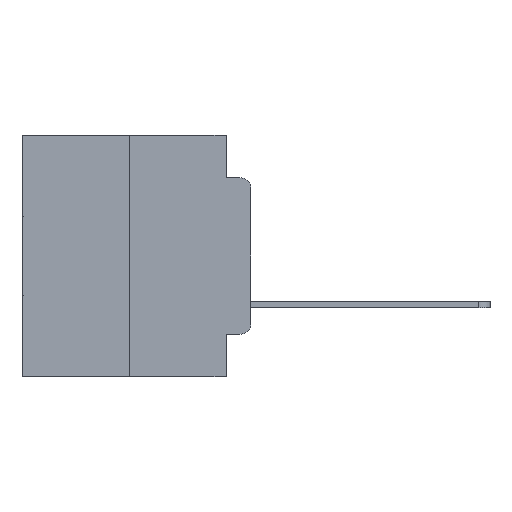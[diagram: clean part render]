
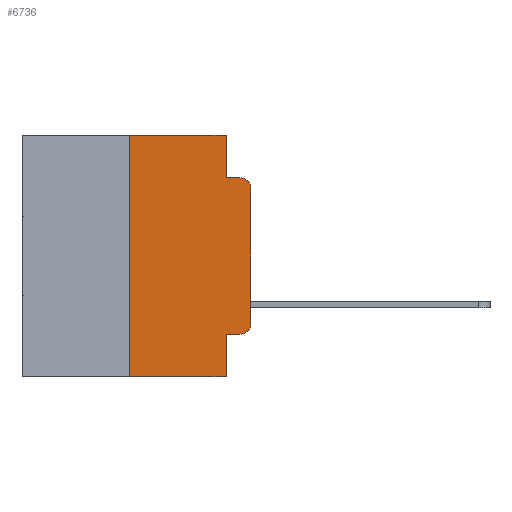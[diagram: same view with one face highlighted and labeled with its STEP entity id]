
A CAD part, left-side view. The second image highlights one B-rep face of the part: STEP entity #6736.
In plain terms, the highlighted planar face has unit normal (-1, 0, 0).
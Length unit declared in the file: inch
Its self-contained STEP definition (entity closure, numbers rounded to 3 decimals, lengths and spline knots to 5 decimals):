
#84 = ORIENTED_EDGE ( 'NONE', *, *, #25238, .F. ) ;
#494 = EDGE_CURVE ( 'NONE', #27528, #16480, #21956, .T. ) ;
#1018 = CARTESIAN_POINT ( 'NONE',  ( 0., 0.02, -0.0885 ) ) ;
#1661 = EDGE_CURVE ( 'NONE', #21829, #10695, #11175, .T. ) ;
#1906 = LINE ( 'NONE', #11384, #2932 ) ;
#2286 = EDGE_LOOP ( 'NONE', ( #9304, #26170, #3473, #11589, #12867, #13742, #19605, #84, #2298, #19662 ) ) ;
#2298 = ORIENTED_EDGE ( 'NONE', *, *, #1661, .T. ) ;
#2320 = LINE ( 'NONE', #20748, #25140 ) ;
#2638 = DIRECTION ( 'NONE',  ( 0., 0., -1. ) ) ;
#2652 = LINE ( 'NONE', #13312, #23407 ) ;
#2932 = VECTOR ( 'NONE', #2638, 39.37008 ) ;
#3473 = ORIENTED_EDGE ( 'NONE', *, *, #16525, .F. ) ;
#3778 = EDGE_CURVE ( 'NONE', #10695, #13114, #21313, .T. ) ;
#4010 = CARTESIAN_POINT ( 'NONE',  ( 0., 0.02, -0.3915 ) ) ;
#4629 = VERTEX_POINT ( 'NONE', #13715 ) ;
#5187 = EDGE_CURVE ( 'NONE', #4629, #9251, #10192, .T. ) ;
#5969 = EDGE_CURVE ( 'NONE', #24840, #12670, #23229, .T. ) ;
#6106 = PLANE ( 'NONE',  #21900 ) ;
#6248 = DIRECTION ( 'NONE',  ( 0., 0., -1. ) ) ;
#6736 = ADVANCED_FACE ( 'NONE', ( #27365 ), #6106, .F. ) ;
#7195 = DIRECTION ( 'NONE',  ( 0., 0., 1. ) ) ;
#7248 = CARTESIAN_POINT ( 'NONE',  ( 0., 0., -0.3915 ) ) ;
#7383 = CARTESIAN_POINT ( 'NONE',  ( 0., 0.25, 0. ) ) ;
#7593 = VECTOR ( 'NONE', #27357, 39.37008 ) ;
#8566 = EDGE_CURVE ( 'NONE', #13114, #27528, #13794, .T. ) ;
#9251 = VERTEX_POINT ( 'NONE', #17275 ) ;
#9286 = AXIS2_PLACEMENT_3D ( 'NONE', #4010, #19790, #6248 ) ;
#9304 = ORIENTED_EDGE ( 'NONE', *, *, #8566, .T. ) ;
#9482 = LINE ( 'NONE', #27719, #25362 ) ;
#9615 = CARTESIAN_POINT ( 'NONE',  ( 0., 0.051, -0.4115 ) ) ;
#10192 = LINE ( 'NONE', #17150, #15701 ) ;
#10695 = VERTEX_POINT ( 'NONE', #22183 ) ;
#11175 = LINE ( 'NONE', #9615, #12557 ) ;
#11384 = CARTESIAN_POINT ( 'NONE',  ( 0., 0.051, 0. ) ) ;
#11589 = ORIENTED_EDGE ( 'NONE', *, *, #5187, .F. ) ;
#12429 = CARTESIAN_POINT ( 'NONE',  ( 0., 0.473, 0. ) ) ;
#12557 = VECTOR ( 'NONE', #22887, 39.37008 ) ;
#12670 = VERTEX_POINT ( 'NONE', #7383 ) ;
#12867 = ORIENTED_EDGE ( 'NONE', *, *, #21327, .F. ) ;
#13114 = VERTEX_POINT ( 'NONE', #7248 ) ;
#13183 = CARTESIAN_POINT ( 'NONE',  ( 0., 0.051, -0.5 ) ) ;
#13290 = CARTESIAN_POINT ( 'NONE',  ( 0., 0.051, -0.4115 ) ) ;
#13312 = CARTESIAN_POINT ( 'NONE',  ( 0., 0.473, 0. ) ) ;
#13608 = AXIS2_PLACEMENT_3D ( 'NONE', #28097, #25869, #27920 ) ;
#13715 = CARTESIAN_POINT ( 'NONE',  ( 0., 0.051, 0. ) ) ;
#13742 = ORIENTED_EDGE ( 'NONE', *, *, #5969, .F. ) ;
#13794 = LINE ( 'NONE', #23200, #7593 ) ;
#15701 = VECTOR ( 'NONE', #25555, 39.37008 ) ;
#16480 = VERTEX_POINT ( 'NONE', #1018 ) ;
#16525 = EDGE_CURVE ( 'NONE', #9251, #16480, #2320, .T. ) ;
#17150 = CARTESIAN_POINT ( 'NONE',  ( 0., 0.051, 0. ) ) ;
#17275 = CARTESIAN_POINT ( 'NONE',  ( 0., 0.051, -0.0885 ) ) ;
#18083 = CARTESIAN_POINT ( 'NONE',  ( 0., 0.25, 0. ) ) ;
#18514 = DIRECTION ( 'NONE',  ( 0., -1., 0. ) ) ;
#18804 = CARTESIAN_POINT ( 'NONE',  ( 0., 0.25, -0.5 ) ) ;
#19152 = DIRECTION ( 'NONE',  ( 0., 0., -1. ) ) ;
#19403 = DIRECTION ( 'NONE',  ( 0., -1., 0. ) ) ;
#19605 = ORIENTED_EDGE ( 'NONE', *, *, #23683, .T. ) ;
#19662 = ORIENTED_EDGE ( 'NONE', *, *, #3778, .T. ) ;
#19790 = DIRECTION ( 'NONE',  ( -1., 0., 0. ) ) ;
#19794 = VECTOR ( 'NONE', #7195, 39.37008 ) ;
#20430 = DIRECTION ( 'NONE',  ( 0., -1., 0. ) ) ;
#20748 = CARTESIAN_POINT ( 'NONE',  ( 0., 0.051, -0.0885 ) ) ;
#21313 = CIRCLE ( 'NONE', #9286, 0.02 ) ;
#21327 = EDGE_CURVE ( 'NONE', #12670, #4629, #2652, .T. ) ;
#21568 = DIRECTION ( 'NONE',  ( 1., 0., 0. ) ) ;
#21829 = VERTEX_POINT ( 'NONE', #13290 ) ;
#21900 = AXIS2_PLACEMENT_3D ( 'NONE', #12429, #21568, #19152 ) ;
#21956 = CIRCLE ( 'NONE', #13608, 0.02 ) ;
#22183 = CARTESIAN_POINT ( 'NONE',  ( 0., 0.02, -0.4115 ) ) ;
#22887 = DIRECTION ( 'NONE',  ( 0., -1., 0. ) ) ;
#23200 = CARTESIAN_POINT ( 'NONE',  ( 0., 0., 0. ) ) ;
#23229 = LINE ( 'NONE', #18083, #19794 ) ;
#23407 = VECTOR ( 'NONE', #20430, 39.37008 ) ;
#23683 = EDGE_CURVE ( 'NONE', #24840, #26201, #9482, .T. ) ;
#24840 = VERTEX_POINT ( 'NONE', #18804 ) ;
#25140 = VECTOR ( 'NONE', #18514, 39.37008 ) ;
#25238 = EDGE_CURVE ( 'NONE', #21829, #26201, #1906, .T. ) ;
#25362 = VECTOR ( 'NONE', #19403, 39.37008 ) ;
#25555 = DIRECTION ( 'NONE',  ( 0., 0., -1. ) ) ;
#25869 = DIRECTION ( 'NONE',  ( -1., 0., 0. ) ) ;
#25996 = CARTESIAN_POINT ( 'NONE',  ( 0., 0., -0.1085 ) ) ;
#26170 = ORIENTED_EDGE ( 'NONE', *, *, #494, .T. ) ;
#26201 = VERTEX_POINT ( 'NONE', #13183 ) ;
#27357 = DIRECTION ( 'NONE',  ( 0., 0., 1. ) ) ;
#27365 = FACE_OUTER_BOUND ( 'NONE', #2286, .T. ) ;
#27528 = VERTEX_POINT ( 'NONE', #25996 ) ;
#27719 = CARTESIAN_POINT ( 'NONE',  ( 0., 0.473, -0.5 ) ) ;
#27920 = DIRECTION ( 'NONE',  ( 0., 0., -1. ) ) ;
#28097 = CARTESIAN_POINT ( 'NONE',  ( 0., 0.02, -0.1085 ) ) ;
